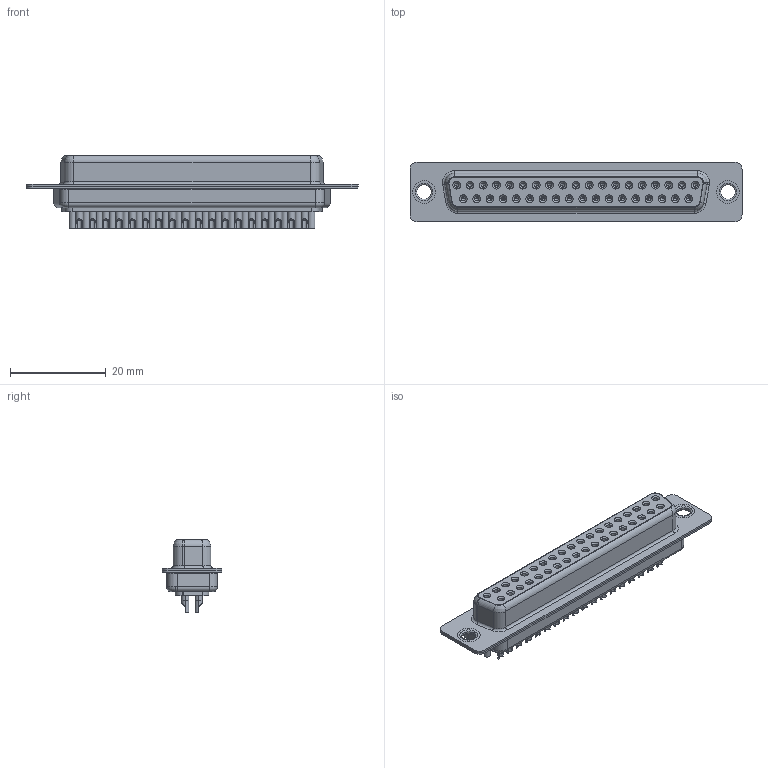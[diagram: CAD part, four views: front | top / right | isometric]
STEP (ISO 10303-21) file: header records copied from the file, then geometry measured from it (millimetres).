
FILE_DESCRIPTION (( 'STEP AP203' ), '1' );
FILE_NAME ('628-M37-322-LT1.STEP', '2021-04-26T14:24:35', ( '' ), ( '' ), 'SwSTEP 2.0', 'SolidWorks 2020', '' );
FILE_SCHEMA (( 'CONFIG_CONTROL_DESIGN' ));
Length unit declared in the file: millimetre
Products named in the file (7): 628M Thru Hole Rivet; 628M Contact Row 2_22; 628M Contact Row 1_22; 628M Housing_37 Contacts; 628-M37-322-LT1; 628M Shell Front_37 Contacts; 628M Shell Rear_37 Contacts
Assembly tree (42 placements, depth 2):
  628-M37-322-LT1
    628M Housing_37 Contacts
    628M Shell Front_37 Contacts
    628M Shell Rear_37 Contacts
    628M Contact Row 1_22  x19
    628M Contact Row 2_22  x18
    628M Thru Hole Rivet  x2
Bounding box: 69.4 x 12.5 x 15.25 mm (x, y, z)
Volume: 5226.6 mm3; surface area: 12815.8 mm2
Topology: 42 solids, 42 shells, 2289 faces, 5635 edges, 3479 vertices
Faces by surface type: cylinder 898, plane 697, torus 361, cone 333
Entity records: 24840 total; most frequent: DIRECTION 4481, CARTESIAN_POINT 4042, ORIENTED_EDGE 3614, AXIS2_PLACEMENT_3D 1896, EDGE_CURVE 1807, VERTEX_POINT 1145, CIRCLE 1052, EDGE_LOOP 1012
